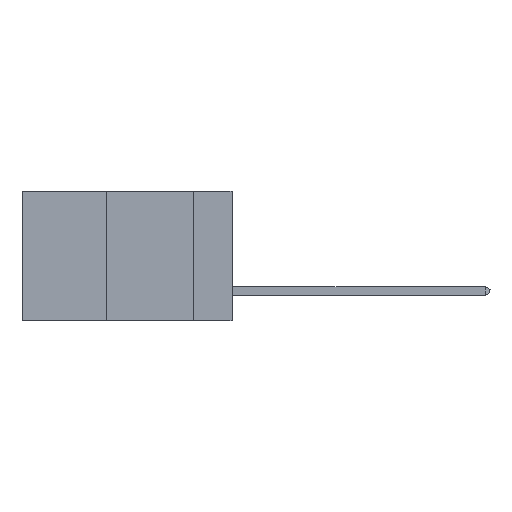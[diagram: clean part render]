
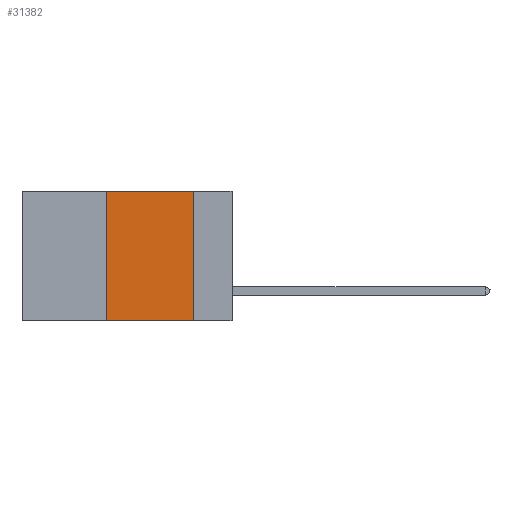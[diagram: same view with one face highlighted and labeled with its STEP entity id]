
A CAD part, left-side view. The second image highlights one B-rep face of the part: STEP entity #31382.
In plain terms, the highlighted planar face has unit normal (-1, 0, 0).
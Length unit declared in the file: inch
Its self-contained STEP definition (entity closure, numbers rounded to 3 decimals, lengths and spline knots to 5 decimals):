
#205 = VECTOR ( 'NONE', #39386, 39.37008 ) ;
#887 = CARTESIAN_POINT ( 'NONE',  ( 0., 0.6, 0. ) ) ;
#1031 = DIRECTION ( 'NONE',  ( 0., 0., -1. ) ) ;
#1385 = LINE ( 'NONE', #41648, #33578 ) ;
#1865 = FACE_OUTER_BOUND ( 'NONE', #31320, .T. ) ;
#5963 = CARTESIAN_POINT ( 'NONE',  ( 0., 0.11, -0.37 ) ) ;
#6245 = ORIENTED_EDGE ( 'NONE', *, *, #30371, .F. ) ;
#9643 = DIRECTION ( 'NONE',  ( 0., -1., 0. ) ) ;
#9705 = CARTESIAN_POINT ( 'NONE',  ( 0., 0.36, -0.37 ) ) ;
#13775 = ORIENTED_EDGE ( 'NONE', *, *, #42678, .T. ) ;
#16320 = CARTESIAN_POINT ( 'NONE',  ( 0., 0.6, -0.37 ) ) ;
#16699 = VECTOR ( 'NONE', #43459, 39.37008 ) ;
#18801 = VERTEX_POINT ( 'NONE', #44996 ) ;
#19098 = CARTESIAN_POINT ( 'NONE',  ( 0., 0.36, 0. ) ) ;
#19670 = ORIENTED_EDGE ( 'NONE', *, *, #39076, .F. ) ;
#19683 = VECTOR ( 'NONE', #9643, 39.37008 ) ;
#20260 = CARTESIAN_POINT ( 'NONE',  ( 0., 0.11, 0. ) ) ;
#21640 = PLANE ( 'NONE',  #35910 ) ;
#22807 = ORIENTED_EDGE ( 'NONE', *, *, #31407, .F. ) ;
#27039 = VERTEX_POINT ( 'NONE', #20260 ) ;
#29281 = DIRECTION ( 'NONE',  ( 1., 0., 0. ) ) ;
#29689 = LINE ( 'NONE', #887, #205 ) ;
#30246 = VERTEX_POINT ( 'NONE', #9705 ) ;
#30371 = EDGE_CURVE ( 'NONE', #27039, #44564, #1385, .T. ) ;
#31194 = DIRECTION ( 'NONE',  ( 0., 0., -1. ) ) ;
#31320 = EDGE_LOOP ( 'NONE', ( #6245, #22807, #19670, #13775 ) ) ;
#31382 = ADVANCED_FACE ( 'NONE', ( #1865 ), #21640, .F. ) ;
#31407 = EDGE_CURVE ( 'NONE', #18801, #27039, #29689, .T. ) ;
#32597 = CARTESIAN_POINT ( 'NONE',  ( 0., 0.6, 0. ) ) ;
#33578 = VECTOR ( 'NONE', #31194, 39.37008 ) ;
#35910 = AXIS2_PLACEMENT_3D ( 'NONE', #32597, #29281, #1031 ) ;
#38503 = LINE ( 'NONE', #19098, #16699 ) ;
#39076 = EDGE_CURVE ( 'NONE', #30246, #18801, #38503, .T. ) ;
#39386 = DIRECTION ( 'NONE',  ( 0., -1., 0. ) ) ;
#40355 = LINE ( 'NONE', #16320, #19683 ) ;
#41648 = CARTESIAN_POINT ( 'NONE',  ( 0., 0.11, 0. ) ) ;
#42678 = EDGE_CURVE ( 'NONE', #30246, #44564, #40355, .T. ) ;
#43459 = DIRECTION ( 'NONE',  ( 0., 0., 1. ) ) ;
#44564 = VERTEX_POINT ( 'NONE', #5963 ) ;
#44996 = CARTESIAN_POINT ( 'NONE',  ( 0., 0.36, 0. ) ) ;
